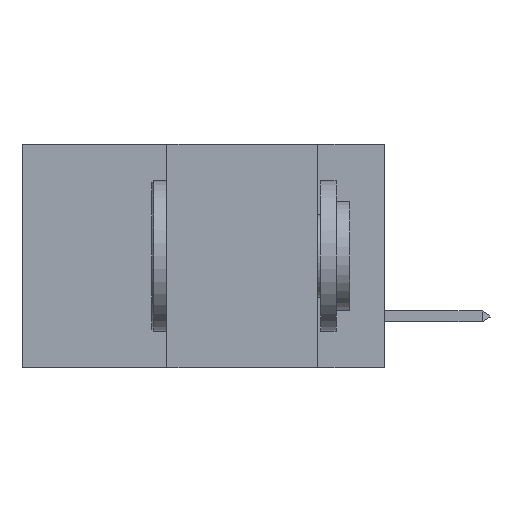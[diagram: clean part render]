
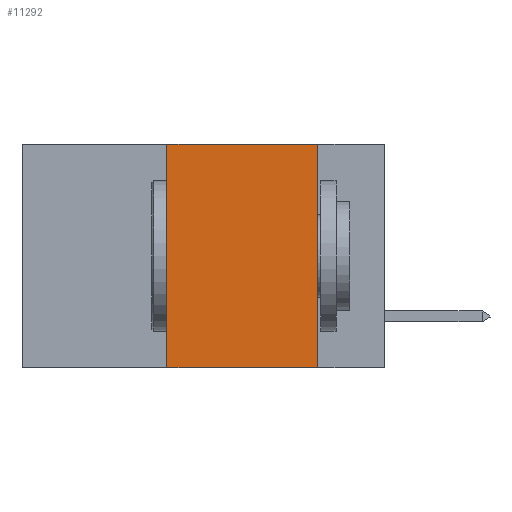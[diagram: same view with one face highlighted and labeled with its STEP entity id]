
A CAD part, left-side view. The second image highlights one B-rep face of the part: STEP entity #11292.
In plain terms, the highlighted planar face has unit normal (-1, 0, 0).
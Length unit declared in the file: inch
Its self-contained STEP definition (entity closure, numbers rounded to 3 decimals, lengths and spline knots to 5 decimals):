
#69 = VERTEX_POINT ( 'NONE', #9874 ) ;
#330 = VECTOR ( 'NONE', #2149, 39.37008 ) ;
#1119 = DIRECTION ( 'NONE',  ( 0., -1., 0. ) ) ;
#1279 = VECTOR ( 'NONE', #11011, 39.37008 ) ;
#2149 = DIRECTION ( 'NONE',  ( 0., 0., 1. ) ) ;
#2178 = LINE ( 'NONE', #8631, #330 ) ;
#2215 = EDGE_CURVE ( 'NONE', #69, #12950, #7521, .T. ) ;
#2289 = CARTESIAN_POINT ( 'NONE',  ( 0., 0.6, -0.37 ) ) ;
#2406 = CARTESIAN_POINT ( 'NONE',  ( 0., 0.6, 0. ) ) ;
#3371 = EDGE_LOOP ( 'NONE', ( #12763, #9321, #9708, #5486 ) ) ;
#4416 = CARTESIAN_POINT ( 'NONE',  ( 0., 0.6, 0. ) ) ;
#5486 = ORIENTED_EDGE ( 'NONE', *, *, #8923, .T. ) ;
#5525 = FACE_OUTER_BOUND ( 'NONE', #3371, .T. ) ;
#6226 = CARTESIAN_POINT ( 'NONE',  ( 0., 0.11, 0. ) ) ;
#6385 = CARTESIAN_POINT ( 'NONE',  ( 0., 0.11, -0.37 ) ) ;
#6633 = DIRECTION ( 'NONE',  ( 1., 0., 0. ) ) ;
#6672 = DIRECTION ( 'NONE',  ( 0., 0., -1. ) ) ;
#7521 = LINE ( 'NONE', #2406, #1279 ) ;
#8216 = CARTESIAN_POINT ( 'NONE',  ( 0., 0.11, 0. ) ) ;
#8631 = CARTESIAN_POINT ( 'NONE',  ( 0., 0.36, 0. ) ) ;
#8746 = DIRECTION ( 'NONE',  ( 0., 0., -1. ) ) ;
#8923 = EDGE_CURVE ( 'NONE', #13491, #10022, #12178, .T. ) ;
#9004 = EDGE_CURVE ( 'NONE', #13491, #69, #2178, .T. ) ;
#9321 = ORIENTED_EDGE ( 'NONE', *, *, #2215, .F. ) ;
#9591 = EDGE_CURVE ( 'NONE', #12950, #10022, #13492, .T. ) ;
#9708 = ORIENTED_EDGE ( 'NONE', *, *, #9004, .F. ) ;
#9874 = CARTESIAN_POINT ( 'NONE',  ( 0., 0.36, 0. ) ) ;
#10022 = VERTEX_POINT ( 'NONE', #6385 ) ;
#10657 = VECTOR ( 'NONE', #6672, 39.37008 ) ;
#10948 = AXIS2_PLACEMENT_3D ( 'NONE', #4416, #6633, #8746 ) ;
#11011 = DIRECTION ( 'NONE',  ( 0., -1., 0. ) ) ;
#11292 = ADVANCED_FACE ( 'NONE', ( #5525 ), #11968, .F. ) ;
#11968 = PLANE ( 'NONE',  #10948 ) ;
#12140 = CARTESIAN_POINT ( 'NONE',  ( 0., 0.36, -0.37 ) ) ;
#12178 = LINE ( 'NONE', #2289, #13851 ) ;
#12763 = ORIENTED_EDGE ( 'NONE', *, *, #9591, .F. ) ;
#12950 = VERTEX_POINT ( 'NONE', #8216 ) ;
#13491 = VERTEX_POINT ( 'NONE', #12140 ) ;
#13492 = LINE ( 'NONE', #6226, #10657 ) ;
#13851 = VECTOR ( 'NONE', #1119, 39.37008 ) ;
